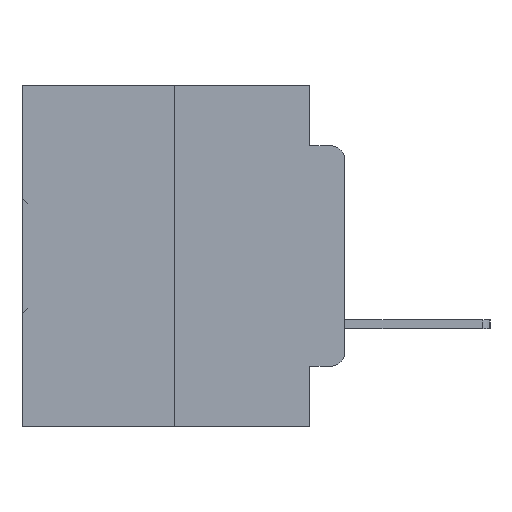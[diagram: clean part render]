
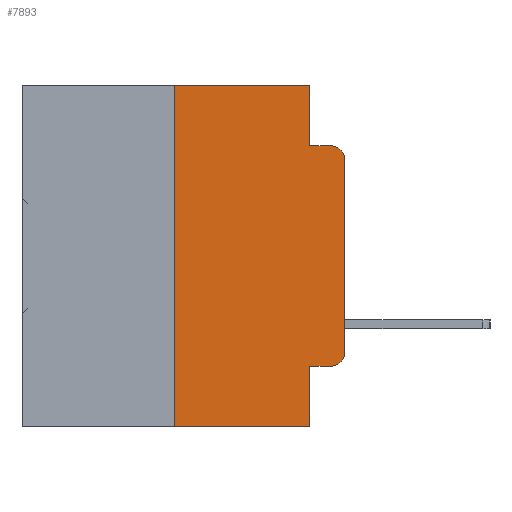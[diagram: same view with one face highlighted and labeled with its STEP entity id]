
A CAD part, left-side view. The second image highlights one B-rep face of the part: STEP entity #7893.
In plain terms, the highlighted planar face has unit normal (-1, 0, 0).
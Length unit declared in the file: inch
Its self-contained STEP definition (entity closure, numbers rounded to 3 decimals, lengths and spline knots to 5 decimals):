
#1071 = CARTESIAN_POINT ( 'NONE',  ( 0., 0.051, -0.5 ) ) ;
#1605 = EDGE_CURVE ( 'NONE', #6293, #29604, #20454, .T. ) ;
#1703 = VERTEX_POINT ( 'NONE', #1071 ) ;
#1719 = EDGE_CURVE ( 'NONE', #13444, #2865, #16406, .T. ) ;
#2197 = CARTESIAN_POINT ( 'NONE',  ( 0., 0.051, 0. ) ) ;
#2240 = VERTEX_POINT ( 'NONE', #32715 ) ;
#2470 = ORIENTED_EDGE ( 'NONE', *, *, #26430, .F. ) ;
#2839 = CARTESIAN_POINT ( 'NONE',  ( 0., 0.25, 0. ) ) ;
#2861 = EDGE_CURVE ( 'NONE', #16422, #13444, #23591, .T. ) ;
#2865 = VERTEX_POINT ( 'NONE', #5301 ) ;
#3433 = ORIENTED_EDGE ( 'NONE', *, *, #19099, .F. ) ;
#3494 = CARTESIAN_POINT ( 'NONE',  ( 0., 0.25, 0. ) ) ;
#5034 = DIRECTION ( 'NONE',  ( 0., -1., 0. ) ) ;
#5301 = CARTESIAN_POINT ( 'NONE',  ( 0., 0.051, -0.0885 ) ) ;
#6257 = DIRECTION ( 'NONE',  ( 0., 0., 1. ) ) ;
#6293 = VERTEX_POINT ( 'NONE', #17619 ) ;
#7697 = ORIENTED_EDGE ( 'NONE', *, *, #31698, .F. ) ;
#7893 = ADVANCED_FACE ( 'NONE', ( #20057 ), #28222, .F. ) ;
#7987 = CIRCLE ( 'NONE', #24671, 0.02 ) ;
#9331 = DIRECTION ( 'NONE',  ( 0., -1., 0. ) ) ;
#9657 = CIRCLE ( 'NONE', #33451, 0.02 ) ;
#9785 = VERTEX_POINT ( 'NONE', #17898 ) ;
#9868 = CARTESIAN_POINT ( 'NONE',  ( 0., 0.02, -0.4115 ) ) ;
#10060 = VECTOR ( 'NONE', #6257, 39.37008 ) ;
#10248 = DIRECTION ( 'NONE',  ( -1., 0., 0. ) ) ;
#10414 = VERTEX_POINT ( 'NONE', #10972 ) ;
#10575 = ORIENTED_EDGE ( 'NONE', *, *, #32613, .T. ) ;
#10972 = CARTESIAN_POINT ( 'NONE',  ( 0., 0., -0.3915 ) ) ;
#11690 = CARTESIAN_POINT ( 'NONE',  ( 0., 0.02, -0.0885 ) ) ;
#11903 = EDGE_CURVE ( 'NONE', #10414, #9785, #31112, .T. ) ;
#12219 = DIRECTION ( 'NONE',  ( -1., 0., 0. ) ) ;
#12248 = DIRECTION ( 'NONE',  ( 0., 0., 1. ) ) ;
#12389 = DIRECTION ( 'NONE',  ( 0., -1., 0. ) ) ;
#12418 = LINE ( 'NONE', #14396, #31854 ) ;
#12457 = VECTOR ( 'NONE', #21208, 39.37008 ) ;
#13444 = VERTEX_POINT ( 'NONE', #2197 ) ;
#13564 = CARTESIAN_POINT ( 'NONE',  ( 0., 0.051, 0. ) ) ;
#14396 = CARTESIAN_POINT ( 'NONE',  ( 0., 0.051, -0.0885 ) ) ;
#15517 = DIRECTION ( 'NONE',  ( 1., 0., 0. ) ) ;
#16190 = ORIENTED_EDGE ( 'NONE', *, *, #1605, .T. ) ;
#16406 = LINE ( 'NONE', #31401, #29920 ) ;
#16422 = VERTEX_POINT ( 'NONE', #2839 ) ;
#17378 = EDGE_CURVE ( 'NONE', #29604, #10414, #7987, .T. ) ;
#17546 = EDGE_CURVE ( 'NONE', #2240, #1703, #23728, .T. ) ;
#17619 = CARTESIAN_POINT ( 'NONE',  ( 0., 0.051, -0.4115 ) ) ;
#17898 = CARTESIAN_POINT ( 'NONE',  ( 0., 0., -0.1085 ) ) ;
#18459 = VECTOR ( 'NONE', #12248, 39.37008 ) ;
#18688 = AXIS2_PLACEMENT_3D ( 'NONE', #30627, #15517, #33231 ) ;
#19035 = ORIENTED_EDGE ( 'NONE', *, *, #2861, .F. ) ;
#19099 = EDGE_CURVE ( 'NONE', #2865, #21801, #12418, .T. ) ;
#19266 = ORIENTED_EDGE ( 'NONE', *, *, #17378, .T. ) ;
#20007 = CARTESIAN_POINT ( 'NONE',  ( 0., 0., 0. ) ) ;
#20057 = FACE_OUTER_BOUND ( 'NONE', #22375, .T. ) ;
#20454 = LINE ( 'NONE', #23970, #33037 ) ;
#20674 = CARTESIAN_POINT ( 'NONE',  ( 0., 0.473, 0. ) ) ;
#21208 = DIRECTION ( 'NONE',  ( 0., 0., -1. ) ) ;
#21801 = VERTEX_POINT ( 'NONE', #11690 ) ;
#22110 = VECTOR ( 'NONE', #5034, 39.37008 ) ;
#22375 = EDGE_LOOP ( 'NONE', ( #22659, #10575, #3433, #32428, #19035, #7697, #27409, #2470, #16190, #19266 ) ) ;
#22659 = ORIENTED_EDGE ( 'NONE', *, *, #11903, .T. ) ;
#22783 = VECTOR ( 'NONE', #12389, 39.37008 ) ;
#23591 = LINE ( 'NONE', #20674, #22783 ) ;
#23728 = LINE ( 'NONE', #30670, #22110 ) ;
#23970 = CARTESIAN_POINT ( 'NONE',  ( 0., 0.051, -0.4115 ) ) ;
#24671 = AXIS2_PLACEMENT_3D ( 'NONE', #27531, #12219, #30025 ) ;
#25244 = DIRECTION ( 'NONE',  ( 0., 0., -1. ) ) ;
#25625 = CARTESIAN_POINT ( 'NONE',  ( 0., 0.02, -0.1085 ) ) ;
#26430 = EDGE_CURVE ( 'NONE', #6293, #1703, #31887, .T. ) ;
#27409 = ORIENTED_EDGE ( 'NONE', *, *, #17546, .T. ) ;
#27531 = CARTESIAN_POINT ( 'NONE',  ( 0., 0.02, -0.3915 ) ) ;
#28138 = DIRECTION ( 'NONE',  ( 0., 0., -1. ) ) ;
#28222 = PLANE ( 'NONE',  #18688 ) ;
#29604 = VERTEX_POINT ( 'NONE', #9868 ) ;
#29920 = VECTOR ( 'NONE', #25244, 39.37008 ) ;
#30025 = DIRECTION ( 'NONE',  ( 0., 0., -1. ) ) ;
#30412 = LINE ( 'NONE', #3494, #10060 ) ;
#30627 = CARTESIAN_POINT ( 'NONE',  ( 0., 0.473, 0. ) ) ;
#30670 = CARTESIAN_POINT ( 'NONE',  ( 0., 0.473, -0.5 ) ) ;
#31112 = LINE ( 'NONE', #20007, #18459 ) ;
#31401 = CARTESIAN_POINT ( 'NONE',  ( 0., 0.051, 0. ) ) ;
#31698 = EDGE_CURVE ( 'NONE', #2240, #16422, #30412, .T. ) ;
#31854 = VECTOR ( 'NONE', #9331, 39.37008 ) ;
#31887 = LINE ( 'NONE', #13564, #12457 ) ;
#31981 = DIRECTION ( 'NONE',  ( 0., -1., 0. ) ) ;
#32428 = ORIENTED_EDGE ( 'NONE', *, *, #1719, .F. ) ;
#32613 = EDGE_CURVE ( 'NONE', #9785, #21801, #9657, .T. ) ;
#32715 = CARTESIAN_POINT ( 'NONE',  ( 0., 0.25, -0.5 ) ) ;
#33037 = VECTOR ( 'NONE', #31981, 39.37008 ) ;
#33231 = DIRECTION ( 'NONE',  ( 0., 0., -1. ) ) ;
#33451 = AXIS2_PLACEMENT_3D ( 'NONE', #25625, #10248, #28138 ) ;
